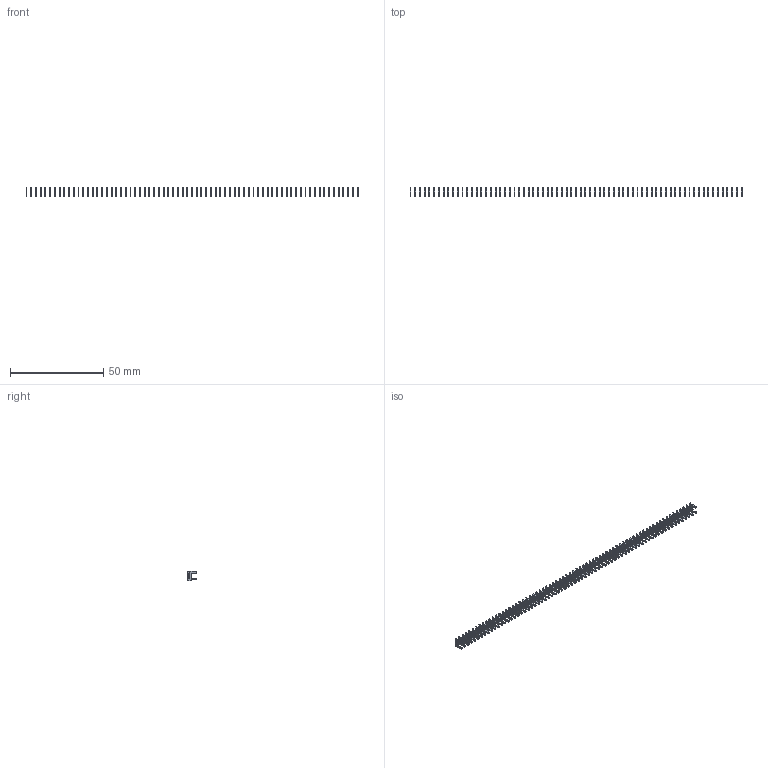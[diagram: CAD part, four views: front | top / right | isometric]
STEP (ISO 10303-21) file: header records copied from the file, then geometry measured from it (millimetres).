
FILE_DESCRIPTION (( 'STEP AP203' ), '1' );
FILE_NAME ('105-071-208-100.STEP', '2020-04-08T01:03:06', ( '' ), ( '' ), 'SwSTEP 2.0', 'SolidWorks 2016', '' );
FILE_SCHEMA (( 'CONFIG_CONTROL_DESIGN' ));
Length unit declared in the file: inch
Products named in the file (2): 100-290-001_100-290-208; 105-071-208-100
Assembly tree (71 placements, depth 2):
  105-071-208-100
    100-290-001_100-290-208  x71
Bounding box: 178.31 x 4.83 x 5.17 mm (x, y, z)
Volume: 488.5 mm3; surface area: 3017.2 mm2
Topology: 71 solids, 71 shells, 1775 faces, 4899 edges, 3266 vertices
Faces by surface type: plane 1562, cylinder 213
Entity records: 3229 total; most frequent: DIRECTION 273, CARTESIAN_POINT 214, COORDINATED_UNIVERSAL_TIME_OFFSET 152, LOCAL_TIME 152, DATE_AND_TIME 152, CALENDAR_DATE 152, ORIENTED_EDGE 138, AXIS2_PLACEMENT_3D 105
